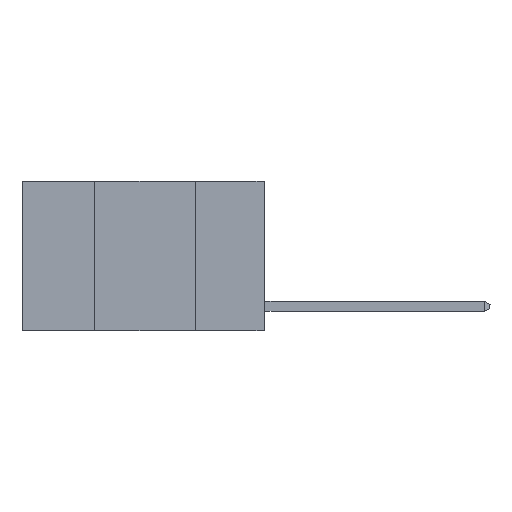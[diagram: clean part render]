
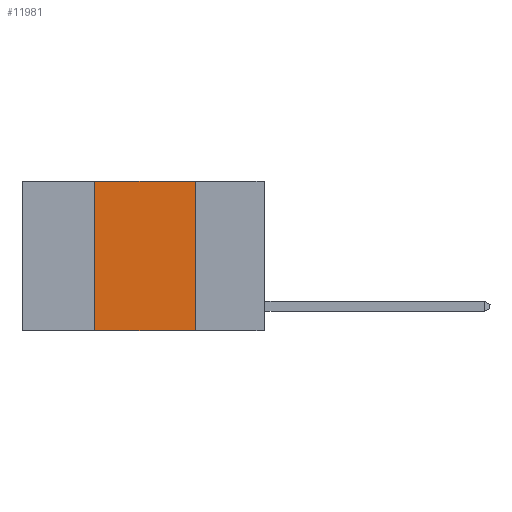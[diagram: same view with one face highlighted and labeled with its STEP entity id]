
A CAD part, left-side view. The second image highlights one B-rep face of the part: STEP entity #11981.
In plain terms, the highlighted planar face has unit normal (-1, 0, 0).
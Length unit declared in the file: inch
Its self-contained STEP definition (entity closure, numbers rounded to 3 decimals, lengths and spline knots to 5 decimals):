
#108 = DIRECTION ( 'NONE',  ( 0., 0., -1. ) ) ;
#554 = CARTESIAN_POINT ( 'NONE',  ( 0., 0.6, -0.37 ) ) ;
#1286 = LINE ( 'NONE', #23404, #16518 ) ;
#2435 = VECTOR ( 'NONE', #19592, 39.37008 ) ;
#2711 = LINE ( 'NONE', #554, #12247 ) ;
#4847 = ORIENTED_EDGE ( 'NONE', *, *, #17173, .F. ) ;
#5203 = EDGE_LOOP ( 'NONE', ( #4847, #16713, #22646, #10929 ) ) ;
#5353 = EDGE_CURVE ( 'NONE', #18665, #22705, #2711, .T. ) ;
#6481 = VERTEX_POINT ( 'NONE', #10858 ) ;
#6601 = CARTESIAN_POINT ( 'NONE',  ( 0., 0.42, -0.37 ) ) ;
#7046 = CARTESIAN_POINT ( 'NONE',  ( 0., 0.6, 0. ) ) ;
#7266 = LINE ( 'NONE', #14637, #21624 ) ;
#9164 = VERTEX_POINT ( 'NONE', #13174 ) ;
#9311 = FACE_OUTER_BOUND ( 'NONE', #5203, .T. ) ;
#10603 = AXIS2_PLACEMENT_3D ( 'NONE', #21964, #16587, #108 ) ;
#10858 = CARTESIAN_POINT ( 'NONE',  ( 0., 0.17, 0. ) ) ;
#10929 = ORIENTED_EDGE ( 'NONE', *, *, #5353, .T. ) ;
#11017 = PLANE ( 'NONE',  #10603 ) ;
#11981 = ADVANCED_FACE ( 'NONE', ( #9311 ), #11017, .F. ) ;
#12247 = VECTOR ( 'NONE', #18965, 39.37008 ) ;
#13174 = CARTESIAN_POINT ( 'NONE',  ( 0., 0.42, 0. ) ) ;
#13788 = CARTESIAN_POINT ( 'NONE',  ( 0., 0.17, -0.37 ) ) ;
#13903 = EDGE_CURVE ( 'NONE', #9164, #6481, #16231, .T. ) ;
#14074 = DIRECTION ( 'NONE',  ( 0., 0., -1. ) ) ;
#14637 = CARTESIAN_POINT ( 'NONE',  ( 0., 0.42, 0. ) ) ;
#16231 = LINE ( 'NONE', #7046, #2435 ) ;
#16518 = VECTOR ( 'NONE', #14074, 39.37008 ) ;
#16587 = DIRECTION ( 'NONE',  ( 1., 0., 0. ) ) ;
#16713 = ORIENTED_EDGE ( 'NONE', *, *, #13903, .F. ) ;
#17173 = EDGE_CURVE ( 'NONE', #6481, #22705, #1286, .T. ) ;
#18665 = VERTEX_POINT ( 'NONE', #6601 ) ;
#18965 = DIRECTION ( 'NONE',  ( 0., -1., 0. ) ) ;
#19592 = DIRECTION ( 'NONE',  ( 0., -1., 0. ) ) ;
#21624 = VECTOR ( 'NONE', #21926, 39.37008 ) ;
#21926 = DIRECTION ( 'NONE',  ( 0., 0., 1. ) ) ;
#21964 = CARTESIAN_POINT ( 'NONE',  ( 0., 0.6, 0. ) ) ;
#22207 = EDGE_CURVE ( 'NONE', #18665, #9164, #7266, .T. ) ;
#22646 = ORIENTED_EDGE ( 'NONE', *, *, #22207, .F. ) ;
#22705 = VERTEX_POINT ( 'NONE', #13788 ) ;
#23404 = CARTESIAN_POINT ( 'NONE',  ( 0., 0.17, 0. ) ) ;
